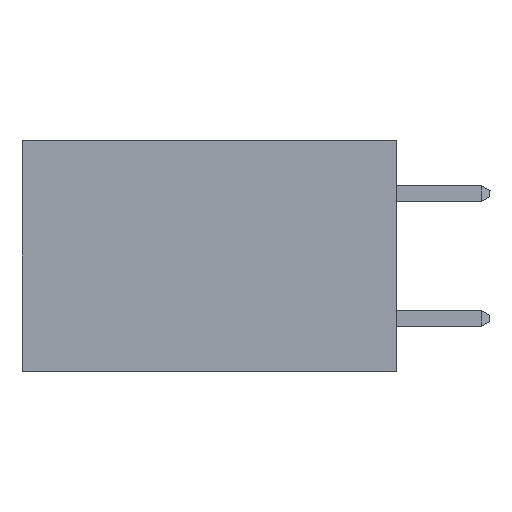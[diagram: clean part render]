
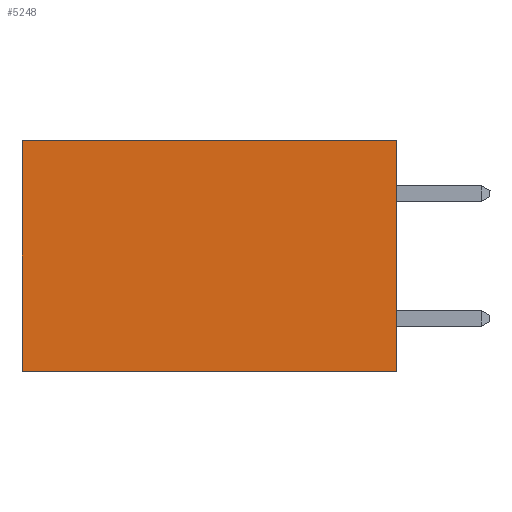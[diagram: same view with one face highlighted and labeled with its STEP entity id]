
A CAD part, left-side view. The second image highlights one B-rep face of the part: STEP entity #5248.
In plain terms, the highlighted planar face has unit normal (-1, 0, 0).
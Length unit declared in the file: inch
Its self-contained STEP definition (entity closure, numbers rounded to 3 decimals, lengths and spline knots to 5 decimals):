
#820 = DIRECTION ( 'NONE',  ( 0., 0., -1. ) ) ;
#885 = VERTEX_POINT ( 'NONE', #5091 ) ;
#1997 = CARTESIAN_POINT ( 'NONE',  ( 0.298, 0.6, 0. ) ) ;
#2187 = LINE ( 'NONE', #7497, #15252 ) ;
#2423 = FACE_OUTER_BOUND ( 'NONE', #6252, .T. ) ;
#2547 = VERTEX_POINT ( 'NONE', #7202 ) ;
#2769 = LINE ( 'NONE', #9288, #14849 ) ;
#4507 = VERTEX_POINT ( 'NONE', #5321 ) ;
#5002 = EDGE_CURVE ( 'NONE', #2547, #8557, #2187, .T. ) ;
#5091 = CARTESIAN_POINT ( 'NONE',  ( 0.298, 0.6, -0.37 ) ) ;
#5248 = ADVANCED_FACE ( 'NONE', ( #2423 ), #17878, .F. ) ;
#5321 = CARTESIAN_POINT ( 'NONE',  ( 0.298, 0., -0.37 ) ) ;
#5666 = CARTESIAN_POINT ( 'NONE',  ( 0.298, 0., 0. ) ) ;
#6252 = EDGE_LOOP ( 'NONE', ( #19099, #7727, #16536, #8638 ) ) ;
#6811 = EDGE_CURVE ( 'NONE', #4507, #885, #2769, .T. ) ;
#7202 = CARTESIAN_POINT ( 'NONE',  ( 0.298, 0., 0. ) ) ;
#7497 = CARTESIAN_POINT ( 'NONE',  ( 0.298, 0., 0. ) ) ;
#7727 = ORIENTED_EDGE ( 'NONE', *, *, #6811, .F. ) ;
#7738 = DIRECTION ( 'NONE',  ( 0., 1., 0. ) ) ;
#8454 = DIRECTION ( 'NONE',  ( 0., 1., 0. ) ) ;
#8509 = CARTESIAN_POINT ( 'NONE',  ( 0.298, 0.6, 0. ) ) ;
#8557 = VERTEX_POINT ( 'NONE', #1997 ) ;
#8638 = ORIENTED_EDGE ( 'NONE', *, *, #5002, .T. ) ;
#9288 = CARTESIAN_POINT ( 'NONE',  ( 0.298, 0., -0.37 ) ) ;
#10174 = DIRECTION ( 'NONE',  ( 0., 0., -1. ) ) ;
#10200 = VECTOR ( 'NONE', #10174, 39.37008 ) ;
#10412 = EDGE_CURVE ( 'NONE', #2547, #4507, #14493, .T. ) ;
#12469 = AXIS2_PLACEMENT_3D ( 'NONE', #13619, #13688, #820 ) ;
#13619 = CARTESIAN_POINT ( 'NONE',  ( 0.298, 0., 0. ) ) ;
#13688 = DIRECTION ( 'NONE',  ( 1., 0., 0. ) ) ;
#14020 = VECTOR ( 'NONE', #15116, 39.37008 ) ;
#14493 = LINE ( 'NONE', #5666, #14020 ) ;
#14849 = VECTOR ( 'NONE', #7738, 39.37008 ) ;
#14870 = LINE ( 'NONE', #8509, #10200 ) ;
#15116 = DIRECTION ( 'NONE',  ( 0., 0., -1. ) ) ;
#15252 = VECTOR ( 'NONE', #8454, 39.37008 ) ;
#16536 = ORIENTED_EDGE ( 'NONE', *, *, #10412, .F. ) ;
#17279 = EDGE_CURVE ( 'NONE', #8557, #885, #14870, .T. ) ;
#17878 = PLANE ( 'NONE',  #12469 ) ;
#19099 = ORIENTED_EDGE ( 'NONE', *, *, #17279, .T. ) ;
